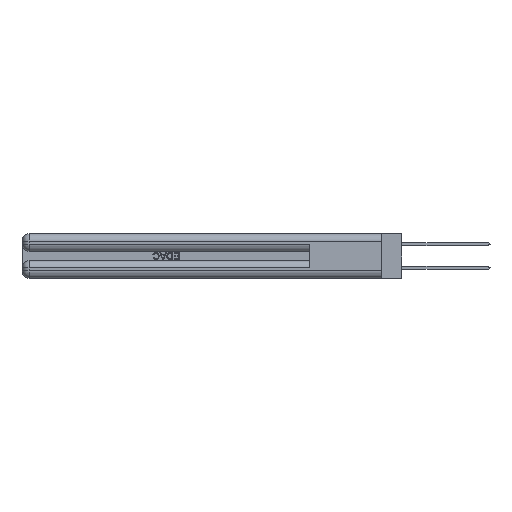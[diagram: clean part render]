
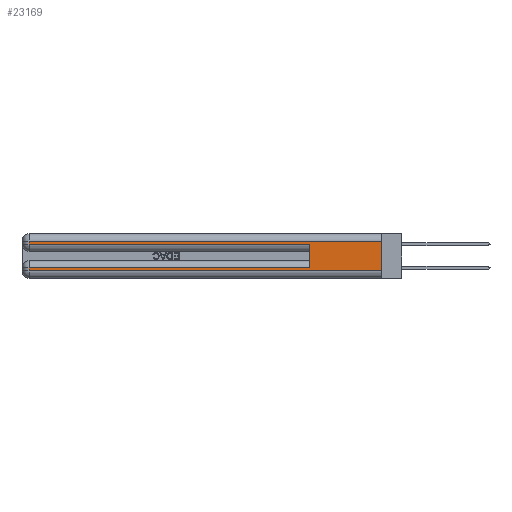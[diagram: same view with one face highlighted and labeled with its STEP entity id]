
A CAD part, left-side view. The second image highlights one B-rep face of the part: STEP entity #23169.
In plain terms, the highlighted planar face has unit normal (-1, 0, 0).
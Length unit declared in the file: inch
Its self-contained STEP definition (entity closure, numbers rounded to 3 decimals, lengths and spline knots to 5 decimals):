
#341 = DIRECTION ( 'NONE',  ( 0., 0., -1. ) ) ;
#2141 = LINE ( 'NONE', #45018, #40476 ) ;
#3078 = CARTESIAN_POINT ( 'NONE',  ( 0., 0.6, 0.145 ) ) ;
#3487 = CARTESIAN_POINT ( 'NONE',  ( 0., 0., 0.085 ) ) ;
#4528 = CARTESIAN_POINT ( 'NONE',  ( 0., 0., 0.37 ) ) ;
#4838 = LINE ( 'NONE', #41091, #24592 ) ;
#5434 = ORIENTED_EDGE ( 'NONE', *, *, #19010, .F. ) ;
#5465 = VECTOR ( 'NONE', #341, 39.37008 ) ;
#6155 = LINE ( 'NONE', #3487, #14896 ) ;
#7612 = CARTESIAN_POINT ( 'NONE',  ( 0., 0., 0.06 ) ) ;
#8090 = EDGE_CURVE ( 'NONE', #20133, #20913, #44941, .T. ) ;
#8147 = ORIENTED_EDGE ( 'NONE', *, *, #36565, .T. ) ;
#8598 = VECTOR ( 'NONE', #20148, 39.37008 ) ;
#8644 = LINE ( 'NONE', #7612, #27233 ) ;
#10531 = DIRECTION ( 'NONE',  ( 0., 0., 1. ) ) ;
#10712 = AXIS2_PLACEMENT_3D ( 'NONE', #10986, #18501, #44417 ) ;
#10986 = CARTESIAN_POINT ( 'NONE',  ( 0., 0., 0.37 ) ) ;
#11346 = DIRECTION ( 'NONE',  ( 0., -1., 0. ) ) ;
#11961 = EDGE_CURVE ( 'NONE', #20913, #38979, #8644, .T. ) ;
#12089 = EDGE_CURVE ( 'NONE', #48027, #38979, #22624, .T. ) ;
#12785 = EDGE_CURVE ( 'NONE', #48027, #45548, #2141, .T. ) ;
#13716 = CARTESIAN_POINT ( 'NONE',  ( 0., 2.94, 0.085 ) ) ;
#14896 = VECTOR ( 'NONE', #33158, 39.37008 ) ;
#16041 = ORIENTED_EDGE ( 'NONE', *, *, #12089, .F. ) ;
#17294 = EDGE_LOOP ( 'NONE', ( #16041, #31742, #44158, #8147, #5434, #32350, #21900, #35986 ) ) ;
#18021 = CARTESIAN_POINT ( 'NONE',  ( 0., 0., 0.06 ) ) ;
#18501 = DIRECTION ( 'NONE',  ( 1., 0., 0. ) ) ;
#18926 = DIRECTION ( 'NONE',  ( 0., 0., -1. ) ) ;
#19010 = EDGE_CURVE ( 'NONE', #33480, #46133, #34728, .T. ) ;
#20133 = VERTEX_POINT ( 'NONE', #13716 ) ;
#20148 = DIRECTION ( 'NONE',  ( 0., -1., 0. ) ) ;
#20913 = VERTEX_POINT ( 'NONE', #44176 ) ;
#21010 = EDGE_CURVE ( 'NONE', #45548, #34737, #4838, .T. ) ;
#21900 = ORIENTED_EDGE ( 'NONE', *, *, #8090, .T. ) ;
#22624 = LINE ( 'NONE', #4528, #31258 ) ;
#23169 = ADVANCED_FACE ( 'NONE', ( #38852 ), #40680, .F. ) ;
#23734 = VECTOR ( 'NONE', #10531, 39.37008 ) ;
#24592 = VECTOR ( 'NONE', #18926, 39.37008 ) ;
#24973 = CARTESIAN_POINT ( 'NONE',  ( 0., 2.94, 0.285 ) ) ;
#26349 = CARTESIAN_POINT ( 'NONE',  ( 0., 2.94, 0.37 ) ) ;
#27233 = VECTOR ( 'NONE', #11346, 39.37008 ) ;
#29763 = CARTESIAN_POINT ( 'NONE',  ( 0., 0.6, 0.285 ) ) ;
#31258 = VECTOR ( 'NONE', #37933, 39.37008 ) ;
#31742 = ORIENTED_EDGE ( 'NONE', *, *, #12785, .T. ) ;
#32350 = ORIENTED_EDGE ( 'NONE', *, *, #42401, .T. ) ;
#32846 = CARTESIAN_POINT ( 'NONE',  ( 0., 0., 0.31 ) ) ;
#33158 = DIRECTION ( 'NONE',  ( 0., 1., 0. ) ) ;
#33480 = VERTEX_POINT ( 'NONE', #38235 ) ;
#34728 = LINE ( 'NONE', #3078, #23734 ) ;
#34737 = VERTEX_POINT ( 'NONE', #24973 ) ;
#35986 = ORIENTED_EDGE ( 'NONE', *, *, #11961, .T. ) ;
#36565 = EDGE_CURVE ( 'NONE', #34737, #46133, #46898, .T. ) ;
#37719 = DIRECTION ( 'NONE',  ( 0., 1., 0. ) ) ;
#37933 = DIRECTION ( 'NONE',  ( 0., 0., -1. ) ) ;
#38235 = CARTESIAN_POINT ( 'NONE',  ( 0., 0.6, 0.085 ) ) ;
#38852 = FACE_OUTER_BOUND ( 'NONE', #17294, .T. ) ;
#38979 = VERTEX_POINT ( 'NONE', #18021 ) ;
#39473 = CARTESIAN_POINT ( 'NONE',  ( 0., 2.94, 0.31 ) ) ;
#40476 = VECTOR ( 'NONE', #37719, 39.37008 ) ;
#40680 = PLANE ( 'NONE',  #10712 ) ;
#41091 = CARTESIAN_POINT ( 'NONE',  ( 0., 2.94, 0.37 ) ) ;
#42401 = EDGE_CURVE ( 'NONE', #33480, #20133, #6155, .T. ) ;
#44158 = ORIENTED_EDGE ( 'NONE', *, *, #21010, .T. ) ;
#44176 = CARTESIAN_POINT ( 'NONE',  ( 0., 2.94, 0.06 ) ) ;
#44417 = DIRECTION ( 'NONE',  ( 0., 0., -1. ) ) ;
#44941 = LINE ( 'NONE', #26349, #5465 ) ;
#45018 = CARTESIAN_POINT ( 'NONE',  ( 0., 0., 0.31 ) ) ;
#45548 = VERTEX_POINT ( 'NONE', #39473 ) ;
#46052 = CARTESIAN_POINT ( 'NONE',  ( 0., 0., 0.285 ) ) ;
#46133 = VERTEX_POINT ( 'NONE', #29763 ) ;
#46898 = LINE ( 'NONE', #46052, #8598 ) ;
#48027 = VERTEX_POINT ( 'NONE', #32846 ) ;
